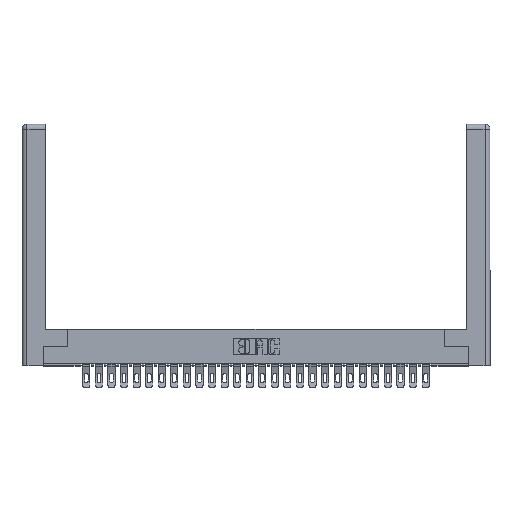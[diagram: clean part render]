
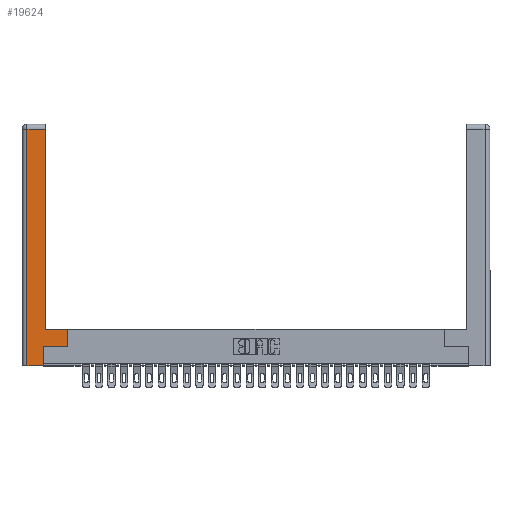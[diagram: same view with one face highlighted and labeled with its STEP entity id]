
A CAD part, top view. The second image highlights one B-rep face of the part: STEP entity #19624.
In plain terms, the highlighted planar face has unit normal (0, 0, 1).
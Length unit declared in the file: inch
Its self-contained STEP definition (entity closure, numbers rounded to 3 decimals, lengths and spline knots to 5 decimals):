
#834 = EDGE_CURVE ( 'NONE', #28183, #24883, #32974, .T. ) ;
#940 = VECTOR ( 'NONE', #1138, 39.37008 ) ;
#1138 = DIRECTION ( 'NONE',  ( 1., 0., 0. ) ) ;
#1771 = FACE_OUTER_BOUND ( 'NONE', #17130, .T. ) ;
#2177 = DIRECTION ( 'NONE',  ( 1., 0., 0. ) ) ;
#2409 = VERTEX_POINT ( 'NONE', #30730 ) ;
#2594 = VERTEX_POINT ( 'NONE', #13532 ) ;
#2781 = CARTESIAN_POINT ( 'NONE',  ( 0.265, 0.245, 0. ) ) ;
#3309 = LINE ( 'NONE', #27475, #26269 ) ;
#3745 = EDGE_CURVE ( 'NONE', #18990, #2409, #23811, .T. ) ;
#4205 = ORIENTED_EDGE ( 'NONE', *, *, #15000, .T. ) ;
#4755 = LINE ( 'NONE', #7756, #17917 ) ;
#6319 = LINE ( 'NONE', #2781, #29293 ) ;
#6400 = CARTESIAN_POINT ( 'NONE',  ( 0.265, 0., 0. ) ) ;
#7756 = CARTESIAN_POINT ( 'NONE',  ( 0.295, 3., 0. ) ) ;
#8164 = DIRECTION ( 'NONE',  ( 0., 0., -1. ) ) ;
#9297 = CARTESIAN_POINT ( 'NONE',  ( 0.0615, 0., 0. ) ) ;
#9808 = EDGE_CURVE ( 'NONE', #31485, #2594, #30288, .T. ) ;
#9963 = EDGE_CURVE ( 'NONE', #10871, #18990, #16237, .T. ) ;
#10443 = CARTESIAN_POINT ( 'NONE',  ( 0.0615, 2.94, 0. ) ) ;
#10467 = DIRECTION ( 'NONE',  ( 0., 1., 0. ) ) ;
#10871 = VERTEX_POINT ( 'NONE', #32563 ) ;
#11179 = CARTESIAN_POINT ( 'NONE',  ( 0.265, 0.245, 0. ) ) ;
#11720 = CARTESIAN_POINT ( 'NONE',  ( 0.565, 0.245, 0. ) ) ;
#12170 = CARTESIAN_POINT ( 'NONE',  ( 0.0615, 2.94, 0. ) ) ;
#12421 = CARTESIAN_POINT ( 'NONE',  ( 0.565, 0.45, 0. ) ) ;
#13170 = VECTOR ( 'NONE', #25912, 39.37008 ) ;
#13532 = CARTESIAN_POINT ( 'NONE',  ( 0.565, 0.245, 0. ) ) ;
#14416 = ORIENTED_EDGE ( 'NONE', *, *, #15162, .T. ) ;
#14792 = EDGE_CURVE ( 'NONE', #15942, #31485, #6319, .T. ) ;
#15000 = EDGE_CURVE ( 'NONE', #2409, #15942, #16065, .T. ) ;
#15162 = EDGE_CURVE ( 'NONE', #2594, #28183, #3309, .T. ) ;
#15942 = VERTEX_POINT ( 'NONE', #6400 ) ;
#16065 = LINE ( 'NONE', #35117, #32271 ) ;
#16118 = PLANE ( 'NONE',  #24030 ) ;
#16202 = ORIENTED_EDGE ( 'NONE', *, *, #25525, .T. ) ;
#16236 = DIRECTION ( 'NONE',  ( -1., 0., 0. ) ) ;
#16237 = LINE ( 'NONE', #12170, #23470 ) ;
#16342 = CARTESIAN_POINT ( 'NONE',  ( 0., 0., 0. ) ) ;
#16536 = ORIENTED_EDGE ( 'NONE', *, *, #9808, .T. ) ;
#17130 = EDGE_LOOP ( 'NONE', ( #16202, #21934, #34502, #4205, #23435, #16536, #14416, #34023 ) ) ;
#17616 = VECTOR ( 'NONE', #29714, 39.37008 ) ;
#17917 = VECTOR ( 'NONE', #10467, 39.37008 ) ;
#18990 = VERTEX_POINT ( 'NONE', #10443 ) ;
#19624 = ADVANCED_FACE ( 'NONE', ( #1771 ), #16118, .F. ) ;
#20588 = CARTESIAN_POINT ( 'NONE',  ( 0.295, 0.45, 0. ) ) ;
#21934 = ORIENTED_EDGE ( 'NONE', *, *, #9963, .T. ) ;
#23435 = ORIENTED_EDGE ( 'NONE', *, *, #14792, .T. ) ;
#23470 = VECTOR ( 'NONE', #33714, 39.37008 ) ;
#23811 = LINE ( 'NONE', #9297, #13170 ) ;
#24030 = AXIS2_PLACEMENT_3D ( 'NONE', #16342, #8164, #16236 ) ;
#24485 = DIRECTION ( 'NONE',  ( 0., 1., 0. ) ) ;
#24883 = VERTEX_POINT ( 'NONE', #20588 ) ;
#25525 = EDGE_CURVE ( 'NONE', #24883, #10871, #4755, .T. ) ;
#25912 = DIRECTION ( 'NONE',  ( 0., -1., 0. ) ) ;
#26269 = VECTOR ( 'NONE', #24485, 39.37008 ) ;
#27475 = CARTESIAN_POINT ( 'NONE',  ( 0.565, 0.45, 0. ) ) ;
#28183 = VERTEX_POINT ( 'NONE', #12421 ) ;
#29293 = VECTOR ( 'NONE', #32513, 39.37008 ) ;
#29714 = DIRECTION ( 'NONE',  ( -1., 0., 0. ) ) ;
#30288 = LINE ( 'NONE', #11720, #940 ) ;
#30730 = CARTESIAN_POINT ( 'NONE',  ( 0.0615, 0., 0. ) ) ;
#31485 = VERTEX_POINT ( 'NONE', #11179 ) ;
#32271 = VECTOR ( 'NONE', #2177, 39.37008 ) ;
#32359 = CARTESIAN_POINT ( 'NONE',  ( 0.295, 0.45, 0. ) ) ;
#32513 = DIRECTION ( 'NONE',  ( 0., 1., 0. ) ) ;
#32563 = CARTESIAN_POINT ( 'NONE',  ( 0.295, 2.94, 0. ) ) ;
#32974 = LINE ( 'NONE', #32359, #17616 ) ;
#33714 = DIRECTION ( 'NONE',  ( -1., 0., 0. ) ) ;
#34023 = ORIENTED_EDGE ( 'NONE', *, *, #834, .T. ) ;
#34502 = ORIENTED_EDGE ( 'NONE', *, *, #3745, .T. ) ;
#35117 = CARTESIAN_POINT ( 'NONE',  ( 0.265, 0., 0. ) ) ;
